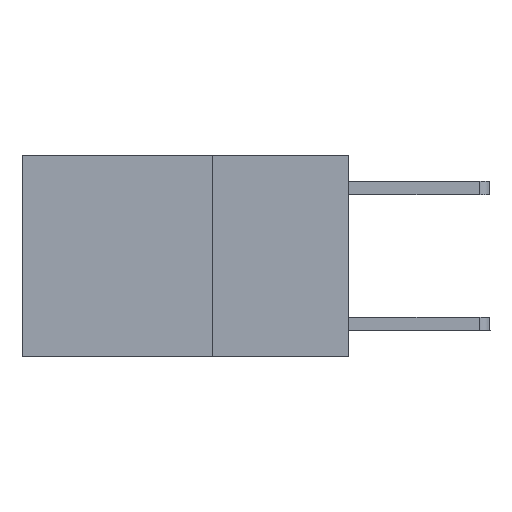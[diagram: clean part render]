
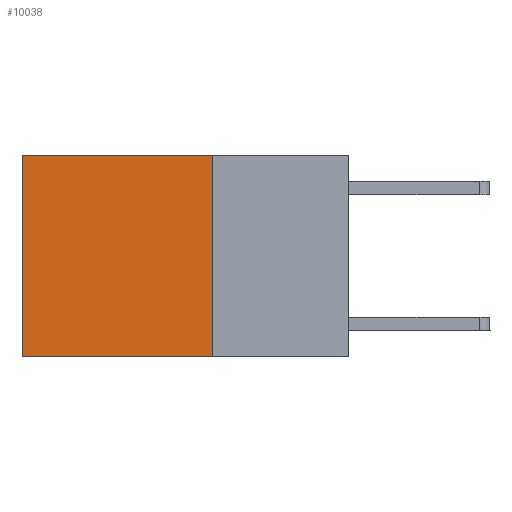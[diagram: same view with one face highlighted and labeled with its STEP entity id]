
A CAD part, left-side view. The second image highlights one B-rep face of the part: STEP entity #10038.
In plain terms, the highlighted planar face has unit normal (-1, 0, 0).
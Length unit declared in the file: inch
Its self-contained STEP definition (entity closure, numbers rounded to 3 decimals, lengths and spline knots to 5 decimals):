
#25 = VECTOR ( 'NONE', #4496, 39.37008 ) ;
#39 = LINE ( 'NONE', #1212, #4758 ) ;
#368 = ORIENTED_EDGE ( 'NONE', *, *, #666, .T. ) ;
#666 = EDGE_CURVE ( 'NONE', #6836, #5491, #3566, .T. ) ;
#1062 = FACE_OUTER_BOUND ( 'NONE', #3534, .T. ) ;
#1212 = CARTESIAN_POINT ( 'NONE',  ( 0.2625, 0.25, 0. ) ) ;
#1339 = CARTESIAN_POINT ( 'NONE',  ( 0.2625, 0.25, 0. ) ) ;
#2921 = EDGE_CURVE ( 'NONE', #7590, #6998, #39, .T. ) ;
#3021 = ORIENTED_EDGE ( 'NONE', *, *, #6113, .F. ) ;
#3295 = CARTESIAN_POINT ( 'NONE',  ( 0.2625, 0.25, 0. ) ) ;
#3438 = EDGE_CURVE ( 'NONE', #7590, #6836, #4501, .T. ) ;
#3534 = EDGE_LOOP ( 'NONE', ( #368, #3021, #6677, #4817 ) ) ;
#3566 = LINE ( 'NONE', #4691, #9567 ) ;
#3813 = AXIS2_PLACEMENT_3D ( 'NONE', #1339, #6454, #8918 ) ;
#4496 = DIRECTION ( 'NONE',  ( 0., 1., 0. ) ) ;
#4501 = LINE ( 'NONE', #9375, #25 ) ;
#4691 = CARTESIAN_POINT ( 'NONE',  ( 0.2625, 0.6, 0. ) ) ;
#4758 = VECTOR ( 'NONE', #7162, 39.37008 ) ;
#4817 = ORIENTED_EDGE ( 'NONE', *, *, #3438, .T. ) ;
#4974 = LINE ( 'NONE', #8293, #8292 ) ;
#5085 = CARTESIAN_POINT ( 'NONE',  ( 0.2625, 0.6, -0.37 ) ) ;
#5491 = VERTEX_POINT ( 'NONE', #5085 ) ;
#5547 = DIRECTION ( 'NONE',  ( 0., 0., -1. ) ) ;
#6113 = EDGE_CURVE ( 'NONE', #6998, #5491, #4974, .T. ) ;
#6454 = DIRECTION ( 'NONE',  ( 1., 0., 0. ) ) ;
#6677 = ORIENTED_EDGE ( 'NONE', *, *, #2921, .F. ) ;
#6714 = CARTESIAN_POINT ( 'NONE',  ( 0.2625, 0.25, -0.37 ) ) ;
#6836 = VERTEX_POINT ( 'NONE', #8135 ) ;
#6998 = VERTEX_POINT ( 'NONE', #6714 ) ;
#7162 = DIRECTION ( 'NONE',  ( 0., 0., -1. ) ) ;
#7590 = VERTEX_POINT ( 'NONE', #3295 ) ;
#8102 = PLANE ( 'NONE',  #3813 ) ;
#8135 = CARTESIAN_POINT ( 'NONE',  ( 0.2625, 0.6, 0. ) ) ;
#8292 = VECTOR ( 'NONE', #10558, 39.37008 ) ;
#8293 = CARTESIAN_POINT ( 'NONE',  ( 0.2625, 0.25, -0.37 ) ) ;
#8918 = DIRECTION ( 'NONE',  ( 0., 0., -1. ) ) ;
#9375 = CARTESIAN_POINT ( 'NONE',  ( 0.2625, 0.25, 0. ) ) ;
#9567 = VECTOR ( 'NONE', #5547, 39.37008 ) ;
#10038 = ADVANCED_FACE ( 'NONE', ( #1062 ), #8102, .F. ) ;
#10558 = DIRECTION ( 'NONE',  ( 0., 1., 0. ) ) ;
